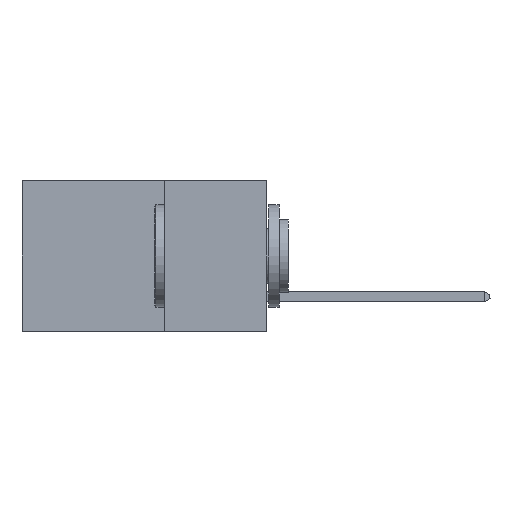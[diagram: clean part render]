
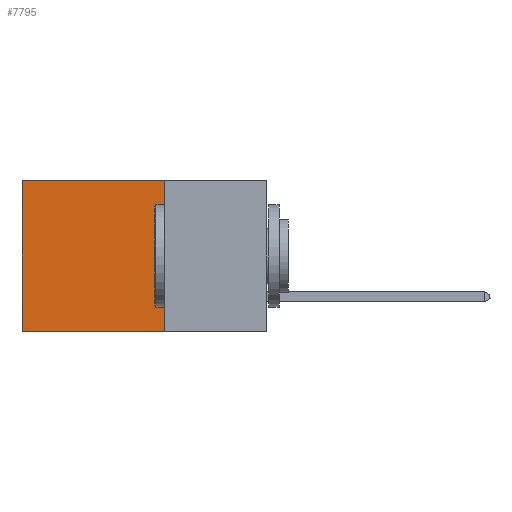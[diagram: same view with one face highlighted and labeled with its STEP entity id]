
A CAD part, left-side view. The second image highlights one B-rep face of the part: STEP entity #7795.
In plain terms, the highlighted planar face has unit normal (-1, 0, 0).
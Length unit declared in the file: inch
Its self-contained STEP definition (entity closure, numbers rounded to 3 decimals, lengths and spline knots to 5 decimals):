
#459 = ORIENTED_EDGE ( 'NONE', *, *, #9245, .T. ) ;
#613 = LINE ( 'NONE', #20911, #17125 ) ;
#740 = LINE ( 'NONE', #14108, #23650 ) ;
#2029 = CARTESIAN_POINT ( 'NONE',  ( 0.2875, 0.6, -0.37 ) ) ;
#2141 = EDGE_CURVE ( 'NONE', #2232, #4792, #14424, .T. ) ;
#2232 = VERTEX_POINT ( 'NONE', #27865 ) ;
#2419 = EDGE_LOOP ( 'NONE', ( #24038, #8833, #17419, #459 ) ) ;
#2729 = FACE_OUTER_BOUND ( 'NONE', #2419, .T. ) ;
#3865 = CARTESIAN_POINT ( 'NONE',  ( 0.2875, 0.25, -0.37 ) ) ;
#4792 = VERTEX_POINT ( 'NONE', #2029 ) ;
#5847 = CARTESIAN_POINT ( 'NONE',  ( 0.2875, 0.6, 0. ) ) ;
#7795 = ADVANCED_FACE ( 'NONE', ( #2729 ), #16700, .F. ) ;
#8085 = DIRECTION ( 'NONE',  ( 0., 1., 0. ) ) ;
#8833 = ORIENTED_EDGE ( 'NONE', *, *, #9831, .F. ) ;
#9245 = EDGE_CURVE ( 'NONE', #27503, #2232, #613, .T. ) ;
#9831 = EDGE_CURVE ( 'NONE', #26855, #4792, #11661, .T. ) ;
#9901 = DIRECTION ( 'NONE',  ( 1., 0., 0. ) ) ;
#11661 = LINE ( 'NONE', #3865, #25530 ) ;
#12247 = CARTESIAN_POINT ( 'NONE',  ( 0.2875, 0.25, 0. ) ) ;
#14108 = CARTESIAN_POINT ( 'NONE',  ( 0.2875, 0.25, 0. ) ) ;
#14424 = LINE ( 'NONE', #5847, #23547 ) ;
#14498 = DIRECTION ( 'NONE',  ( 0., 1., 0. ) ) ;
#16700 = PLANE ( 'NONE',  #19323 ) ;
#16928 = EDGE_CURVE ( 'NONE', #27503, #26855, #740, .T. ) ;
#17125 = VECTOR ( 'NONE', #14498, 39.37008 ) ;
#17419 = ORIENTED_EDGE ( 'NONE', *, *, #16928, .F. ) ;
#19323 = AXIS2_PLACEMENT_3D ( 'NONE', #12247, #9901, #27480 ) ;
#20602 = DIRECTION ( 'NONE',  ( 0., 0., -1. ) ) ;
#20862 = DIRECTION ( 'NONE',  ( 0., 0., -1. ) ) ;
#20911 = CARTESIAN_POINT ( 'NONE',  ( 0.2875, 0.25, 0. ) ) ;
#23547 = VECTOR ( 'NONE', #20862, 39.37008 ) ;
#23650 = VECTOR ( 'NONE', #20602, 39.37008 ) ;
#23885 = CARTESIAN_POINT ( 'NONE',  ( 0.2875, 0.25, -0.37 ) ) ;
#24038 = ORIENTED_EDGE ( 'NONE', *, *, #2141, .T. ) ;
#25530 = VECTOR ( 'NONE', #8085, 39.37008 ) ;
#26295 = CARTESIAN_POINT ( 'NONE',  ( 0.2875, 0.25, 0. ) ) ;
#26855 = VERTEX_POINT ( 'NONE', #23885 ) ;
#27480 = DIRECTION ( 'NONE',  ( 0., 0., -1. ) ) ;
#27503 = VERTEX_POINT ( 'NONE', #26295 ) ;
#27865 = CARTESIAN_POINT ( 'NONE',  ( 0.2875, 0.6, 0. ) ) ;
